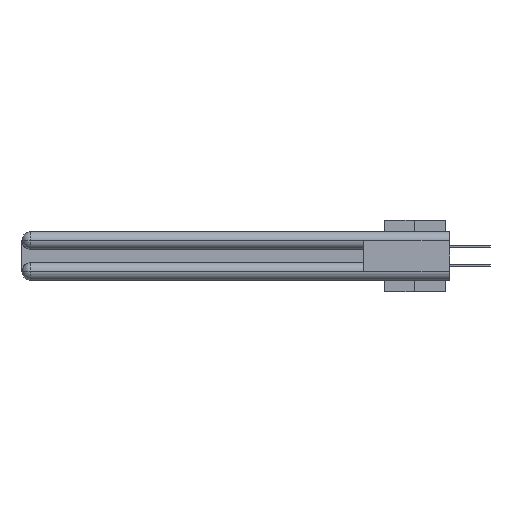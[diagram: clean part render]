
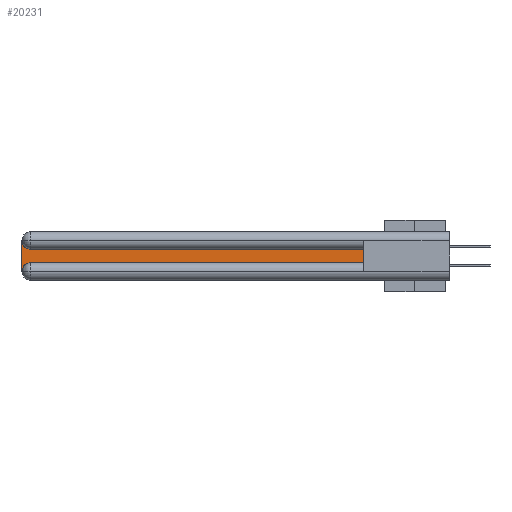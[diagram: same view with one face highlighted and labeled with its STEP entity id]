
A CAD part, left-side view. The second image highlights one B-rep face of the part: STEP entity #20231.
In plain terms, the highlighted planar face has unit normal (-1, 0, 0).
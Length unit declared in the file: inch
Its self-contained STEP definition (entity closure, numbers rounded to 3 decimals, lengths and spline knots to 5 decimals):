
#159 = CARTESIAN_POINT ( 'NONE',  ( 0.075, 2.94, -0.2175 ) ) ;
#1260 = EDGE_CURVE ( 'NONE', #32971, #10491, #47058, .T. ) ;
#2204 = DIRECTION ( 'NONE',  ( 0., 0., 1. ) ) ;
#2622 = CARTESIAN_POINT ( 'NONE',  ( 0.075, 2.94, -0.1225 ) ) ;
#2624 = AXIS2_PLACEMENT_3D ( 'NONE', #29786, #14866, #7551 ) ;
#2686 = EDGE_CURVE ( 'NONE', #32757, #8412, #2741, .T. ) ;
#2689 = FACE_OUTER_BOUND ( 'NONE', #38514, .T. ) ;
#2741 = CIRCLE ( 'NONE', #2624, 0.06 ) ;
#2887 = CARTESIAN_POINT ( 'NONE',  ( 0.075, 3., -0.1225 ) ) ;
#4827 = CIRCLE ( 'NONE', #24128, 0.06 ) ;
#4861 = CARTESIAN_POINT ( 'NONE',  ( 0.075, 0.6, -0.1225 ) ) ;
#5998 = DIRECTION ( 'NONE',  ( 0., -1., 0. ) ) ;
#7551 = DIRECTION ( 'NONE',  ( 0., 0., -1. ) ) ;
#8298 = ORIENTED_EDGE ( 'NONE', *, *, #27018, .T. ) ;
#8412 = VERTEX_POINT ( 'NONE', #44868 ) ;
#9017 = CARTESIAN_POINT ( 'NONE',  ( 0.075, 0.6, -0.2175 ) ) ;
#10037 = DIRECTION ( 'NONE',  ( 0., 0., -1. ) ) ;
#10072 = PLANE ( 'NONE',  #31406 ) ;
#10491 = VERTEX_POINT ( 'NONE', #9017 ) ;
#12935 = ORIENTED_EDGE ( 'NONE', *, *, #22331, .T. ) ;
#13422 = VECTOR ( 'NONE', #5998, 39.37008 ) ;
#13598 = EDGE_CURVE ( 'NONE', #23261, #32971, #4827, .T. ) ;
#14866 = DIRECTION ( 'NONE',  ( 1., 0., 0. ) ) ;
#16816 = LINE ( 'NONE', #35570, #42324 ) ;
#17132 = CARTESIAN_POINT ( 'NONE',  ( 0.075, 2.94, -0.2775 ) ) ;
#18507 = EDGE_CURVE ( 'NONE', #8412, #23261, #34794, .T. ) ;
#18520 = ORIENTED_EDGE ( 'NONE', *, *, #2686, .T. ) ;
#20231 = ADVANCED_FACE ( 'NONE', ( #2689 ), #10072, .F. ) ;
#22331 = EDGE_CURVE ( 'NONE', #10491, #28818, #45497, .T. ) ;
#23261 = VERTEX_POINT ( 'NONE', #26696 ) ;
#24128 = AXIS2_PLACEMENT_3D ( 'NONE', #17132, #28020, #39506 ) ;
#25656 = DIRECTION ( 'NONE',  ( 0., 0., -1. ) ) ;
#26696 = CARTESIAN_POINT ( 'NONE',  ( 0.075, 3., -0.2775 ) ) ;
#27018 = EDGE_CURVE ( 'NONE', #28818, #32757, #16816, .T. ) ;
#27837 = VECTOR ( 'NONE', #2204, 39.37008 ) ;
#28020 = DIRECTION ( 'NONE',  ( 1., 0., 0. ) ) ;
#28068 = CARTESIAN_POINT ( 'NONE',  ( 0.075, 3., -0.2175 ) ) ;
#28818 = VERTEX_POINT ( 'NONE', #4861 ) ;
#29786 = CARTESIAN_POINT ( 'NONE',  ( 0.075, 2.94, -0.0625 ) ) ;
#31406 = AXIS2_PLACEMENT_3D ( 'NONE', #2887, #47361, #25656 ) ;
#32757 = VERTEX_POINT ( 'NONE', #2622 ) ;
#32971 = VERTEX_POINT ( 'NONE', #159 ) ;
#34794 = LINE ( 'NONE', #28068, #46984 ) ;
#35570 = CARTESIAN_POINT ( 'NONE',  ( 0.075, 0.6, -0.1225 ) ) ;
#38514 = EDGE_LOOP ( 'NONE', ( #8298, #18520, #43674, #38909, #45978, #12935 ) ) ;
#38759 = CARTESIAN_POINT ( 'NONE',  ( 0.075, 0.6, -0.2175 ) ) ;
#38909 = ORIENTED_EDGE ( 'NONE', *, *, #13598, .T. ) ;
#39297 = CARTESIAN_POINT ( 'NONE',  ( 0.075, 0.6, -0.2175 ) ) ;
#39506 = DIRECTION ( 'NONE',  ( 0., 0., -1. ) ) ;
#42324 = VECTOR ( 'NONE', #46442, 39.37008 ) ;
#43674 = ORIENTED_EDGE ( 'NONE', *, *, #18507, .T. ) ;
#44868 = CARTESIAN_POINT ( 'NONE',  ( 0.075, 3., -0.0625 ) ) ;
#45497 = LINE ( 'NONE', #38759, #27837 ) ;
#45978 = ORIENTED_EDGE ( 'NONE', *, *, #1260, .T. ) ;
#46442 = DIRECTION ( 'NONE',  ( 0., 1., 0. ) ) ;
#46984 = VECTOR ( 'NONE', #10037, 39.37008 ) ;
#47058 = LINE ( 'NONE', #39297, #13422 ) ;
#47361 = DIRECTION ( 'NONE',  ( 1., 0., 0. ) ) ;
